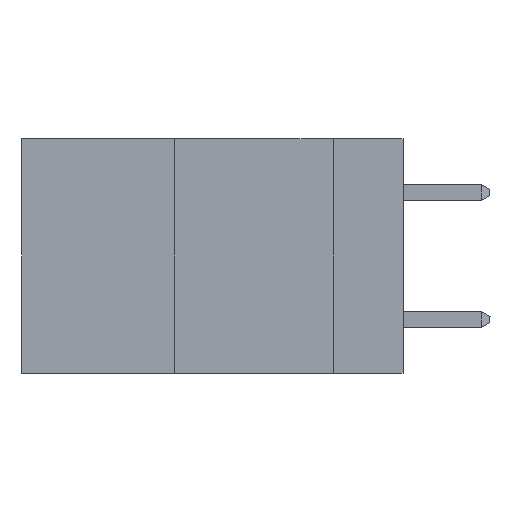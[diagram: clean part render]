
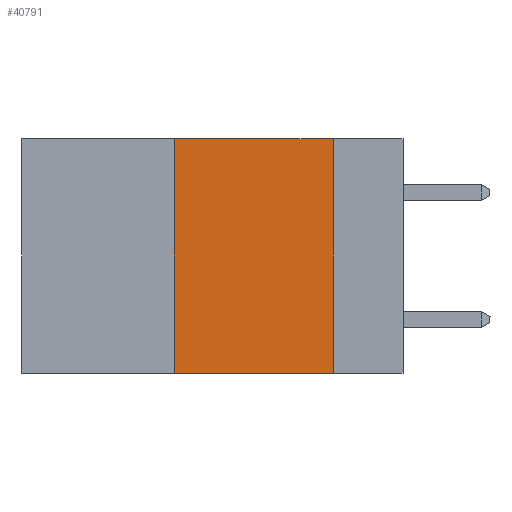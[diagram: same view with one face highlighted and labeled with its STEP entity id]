
A CAD part, left-side view. The second image highlights one B-rep face of the part: STEP entity #40791.
In plain terms, the highlighted planar face has unit normal (-1, 0, 0).
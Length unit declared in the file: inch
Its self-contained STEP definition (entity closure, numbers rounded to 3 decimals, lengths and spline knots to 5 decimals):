
#567 = PLANE ( 'NONE',  #5214 ) ;
#725 = EDGE_CURVE ( 'NONE', #39123, #6351, #38887, .T. ) ;
#877 = LINE ( 'NONE', #11572, #15789 ) ;
#1124 = VERTEX_POINT ( 'NONE', #34447 ) ;
#1200 = VECTOR ( 'NONE', #11837, 39.37008 ) ;
#4757 = CARTESIAN_POINT ( 'NONE',  ( 0., 0.6, 0. ) ) ;
#5214 = AXIS2_PLACEMENT_3D ( 'NONE', #4757, #32856, #39822 ) ;
#6351 = VERTEX_POINT ( 'NONE', #14645 ) ;
#7060 = CARTESIAN_POINT ( 'NONE',  ( 0., 0.6, 0. ) ) ;
#8255 = VECTOR ( 'NONE', #40786, 39.37008 ) ;
#9692 = VECTOR ( 'NONE', #20327, 39.37008 ) ;
#10199 = EDGE_LOOP ( 'NONE', ( #42379, #18130, #13579, #11961 ) ) ;
#11572 = CARTESIAN_POINT ( 'NONE',  ( 0., 0.11, 0. ) ) ;
#11837 = DIRECTION ( 'NONE',  ( 0., 0., 1. ) ) ;
#11961 = ORIENTED_EDGE ( 'NONE', *, *, #30497, .T. ) ;
#13579 = ORIENTED_EDGE ( 'NONE', *, *, #18649, .F. ) ;
#14645 = CARTESIAN_POINT ( 'NONE',  ( 0., 0.11, 0. ) ) ;
#15789 = VECTOR ( 'NONE', #25739, 39.37008 ) ;
#16341 = CARTESIAN_POINT ( 'NONE',  ( 0., 0.11, -0.37 ) ) ;
#16644 = VERTEX_POINT ( 'NONE', #16341 ) ;
#18130 = ORIENTED_EDGE ( 'NONE', *, *, #725, .F. ) ;
#18649 = EDGE_CURVE ( 'NONE', #1124, #39123, #29280, .T. ) ;
#20327 = DIRECTION ( 'NONE',  ( 0., -1., 0. ) ) ;
#20576 = LINE ( 'NONE', #26620, #8255 ) ;
#25739 = DIRECTION ( 'NONE',  ( 0., 0., -1. ) ) ;
#26472 = CARTESIAN_POINT ( 'NONE',  ( 0., 0.36, 0. ) ) ;
#26620 = CARTESIAN_POINT ( 'NONE',  ( 0., 0.6, -0.37 ) ) ;
#29280 = LINE ( 'NONE', #26472, #1200 ) ;
#30497 = EDGE_CURVE ( 'NONE', #1124, #16644, #20576, .T. ) ;
#32408 = FACE_OUTER_BOUND ( 'NONE', #10199, .T. ) ;
#32615 = EDGE_CURVE ( 'NONE', #6351, #16644, #877, .T. ) ;
#32856 = DIRECTION ( 'NONE',  ( 1., 0., 0. ) ) ;
#34447 = CARTESIAN_POINT ( 'NONE',  ( 0., 0.36, -0.37 ) ) ;
#38887 = LINE ( 'NONE', #7060, #9692 ) ;
#39123 = VERTEX_POINT ( 'NONE', #45819 ) ;
#39822 = DIRECTION ( 'NONE',  ( 0., 0., -1. ) ) ;
#40786 = DIRECTION ( 'NONE',  ( 0., -1., 0. ) ) ;
#40791 = ADVANCED_FACE ( 'NONE', ( #32408 ), #567, .F. ) ;
#42379 = ORIENTED_EDGE ( 'NONE', *, *, #32615, .F. ) ;
#45819 = CARTESIAN_POINT ( 'NONE',  ( 0., 0.36, 0. ) ) ;
